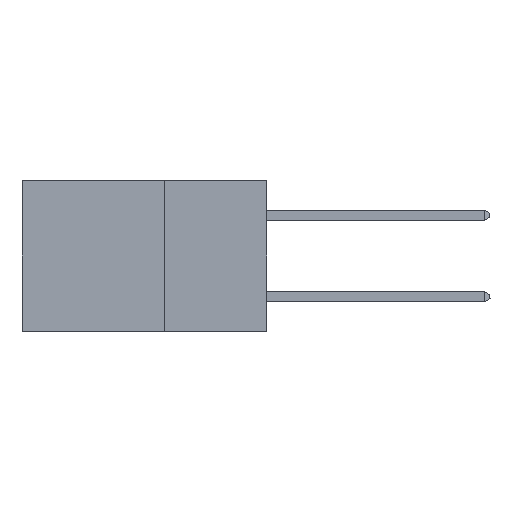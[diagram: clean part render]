
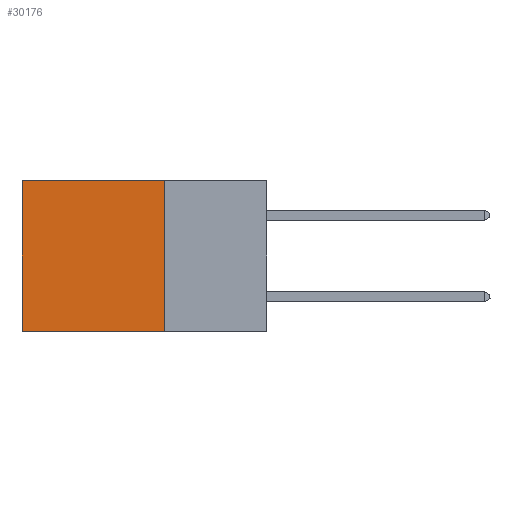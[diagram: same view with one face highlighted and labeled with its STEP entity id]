
A CAD part, left-side view. The second image highlights one B-rep face of the part: STEP entity #30176.
In plain terms, the highlighted planar face has unit normal (-1, 0, 0).
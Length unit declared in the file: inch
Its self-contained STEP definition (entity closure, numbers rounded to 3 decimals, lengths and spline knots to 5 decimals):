
#1474 = CARTESIAN_POINT ( 'NONE',  ( 0.2875, 0.25, 0. ) ) ;
#1498 = LINE ( 'NONE', #26915, #33672 ) ;
#2446 = DIRECTION ( 'NONE',  ( 0., 1., 0. ) ) ;
#3353 = ORIENTED_EDGE ( 'NONE', *, *, #4254, .F. ) ;
#4254 = EDGE_CURVE ( 'NONE', #23776, #10842, #23765, .T. ) ;
#5098 = VECTOR ( 'NONE', #33839, 39.37008 ) ;
#5277 = DIRECTION ( 'NONE',  ( 1., 0., 0. ) ) ;
#8590 = AXIS2_PLACEMENT_3D ( 'NONE', #1474, #5277, #29577 ) ;
#8834 = CARTESIAN_POINT ( 'NONE',  ( 0.2875, 0.25, 0. ) ) ;
#8997 = CARTESIAN_POINT ( 'NONE',  ( 0.2875, 0.25, -0.37 ) ) ;
#9960 = EDGE_CURVE ( 'NONE', #10842, #28358, #41256, .T. ) ;
#10023 = VECTOR ( 'NONE', #2446, 39.37008 ) ;
#10842 = VERTEX_POINT ( 'NONE', #35291 ) ;
#13508 = DIRECTION ( 'NONE',  ( 0., 0., -1. ) ) ;
#14679 = ORIENTED_EDGE ( 'NONE', *, *, #32067, .T. ) ;
#14980 = CARTESIAN_POINT ( 'NONE',  ( 0.2875, 0.6, -0.37 ) ) ;
#19316 = ORIENTED_EDGE ( 'NONE', *, *, #9960, .F. ) ;
#19354 = VECTOR ( 'NONE', #13508, 39.37008 ) ;
#22201 = FACE_OUTER_BOUND ( 'NONE', #29434, .T. ) ;
#23765 = LINE ( 'NONE', #38559, #19354 ) ;
#23776 = VERTEX_POINT ( 'NONE', #8834 ) ;
#25248 = CARTESIAN_POINT ( 'NONE',  ( 0.2875, 0.6, 0. ) ) ;
#26915 = CARTESIAN_POINT ( 'NONE',  ( 0.2875, 0.6, 0. ) ) ;
#28358 = VERTEX_POINT ( 'NONE', #14980 ) ;
#29434 = EDGE_LOOP ( 'NONE', ( #14679, #19316, #3353, #33114 ) ) ;
#29528 = VERTEX_POINT ( 'NONE', #25248 ) ;
#29577 = DIRECTION ( 'NONE',  ( 0., 0., -1. ) ) ;
#30176 = ADVANCED_FACE ( 'NONE', ( #22201 ), #37130, .F. ) ;
#32067 = EDGE_CURVE ( 'NONE', #29528, #28358, #1498, .T. ) ;
#33114 = ORIENTED_EDGE ( 'NONE', *, *, #35993, .T. ) ;
#33672 = VECTOR ( 'NONE', #40938, 39.37008 ) ;
#33839 = DIRECTION ( 'NONE',  ( 0., 1., 0. ) ) ;
#35291 = CARTESIAN_POINT ( 'NONE',  ( 0.2875, 0.25, -0.37 ) ) ;
#35993 = EDGE_CURVE ( 'NONE', #23776, #29528, #40633, .T. ) ;
#37130 = PLANE ( 'NONE',  #8590 ) ;
#38559 = CARTESIAN_POINT ( 'NONE',  ( 0.2875, 0.25, 0. ) ) ;
#40633 = LINE ( 'NONE', #45291, #10023 ) ;
#40938 = DIRECTION ( 'NONE',  ( 0., 0., -1. ) ) ;
#41256 = LINE ( 'NONE', #8997, #5098 ) ;
#45291 = CARTESIAN_POINT ( 'NONE',  ( 0.2875, 0.25, 0. ) ) ;
